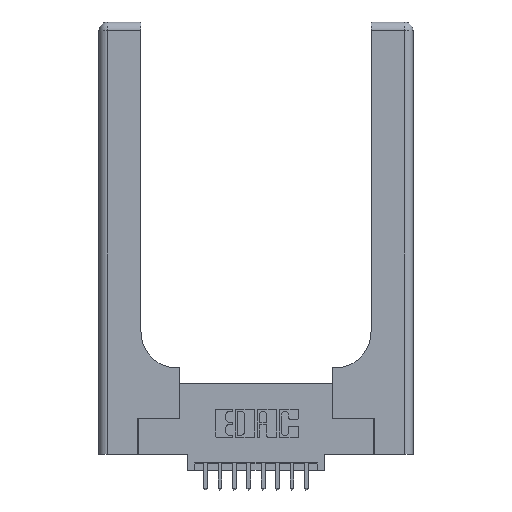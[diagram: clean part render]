
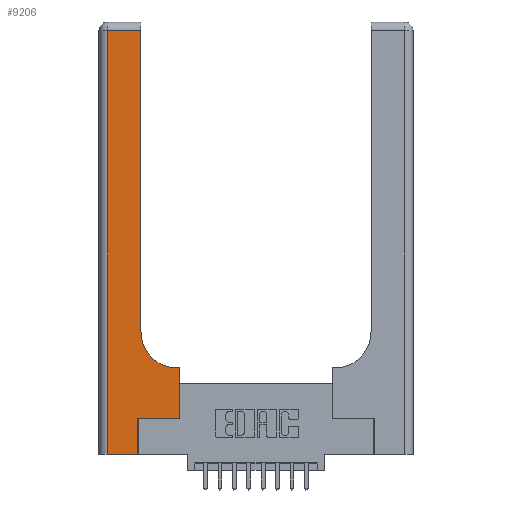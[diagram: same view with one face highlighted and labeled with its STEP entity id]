
A CAD part, top view. The second image highlights one B-rep face of the part: STEP entity #9206.
In plain terms, the highlighted planar face has unit normal (0, 0, 1).
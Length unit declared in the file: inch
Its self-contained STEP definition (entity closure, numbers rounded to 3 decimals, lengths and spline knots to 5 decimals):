
#89 = VERTEX_POINT ( 'NONE', #3098 ) ;
#274 = EDGE_CURVE ( 'NONE', #4211, #10207, #3985, .T. ) ;
#638 = VECTOR ( 'NONE', #4771, 39.37008 ) ;
#781 = LINE ( 'NONE', #11158, #16018 ) ;
#906 = FACE_OUTER_BOUND ( 'NONE', #12245, .T. ) ;
#949 = ORIENTED_EDGE ( 'NONE', *, *, #274, .T. ) ;
#1540 = ORIENTED_EDGE ( 'NONE', *, *, #3682, .T. ) ;
#1818 = DIRECTION ( 'NONE',  ( -1., 0., 0. ) ) ;
#2000 = VECTOR ( 'NONE', #11698, 39.37008 ) ;
#2294 = EDGE_CURVE ( 'NONE', #89, #9336, #5552, .T. ) ;
#2341 = LINE ( 'NONE', #11331, #15813 ) ;
#2592 = LINE ( 'NONE', #10389, #2000 ) ;
#3098 = CARTESIAN_POINT ( 'NONE',  ( 0.06, 2.94, 0.37 ) ) ;
#3407 = VECTOR ( 'NONE', #9392, 39.37008 ) ;
#3682 = EDGE_CURVE ( 'NONE', #9336, #14236, #8058, .T. ) ;
#3825 = CARTESIAN_POINT ( 'NONE',  ( 0.5585, 0.25, 0.37 ) ) ;
#3893 = AXIS2_PLACEMENT_3D ( 'NONE', #16119, #11271, #12535 ) ;
#3985 = CIRCLE ( 'NONE', #3893, 0.25 ) ;
#4026 = CARTESIAN_POINT ( 'NONE',  ( 0.269, 0.25, 0.37 ) ) ;
#4211 = VERTEX_POINT ( 'NONE', #8186 ) ;
#4319 = PLANE ( 'NONE',  #9111 ) ;
#4596 = DIRECTION ( 'NONE',  ( 0., 1., 0. ) ) ;
#4752 = EDGE_CURVE ( 'NONE', #10694, #9421, #10608, .T. ) ;
#4771 = DIRECTION ( 'NONE',  ( 1., 0., 0. ) ) ;
#4929 = CARTESIAN_POINT ( 'NONE',  ( 0.2915, 0.85, 0.37 ) ) ;
#5077 = ORIENTED_EDGE ( 'NONE', *, *, #10045, .T. ) ;
#5552 = LINE ( 'NONE', #13077, #3407 ) ;
#5838 = CARTESIAN_POINT ( 'NONE',  ( 0.5585, 0.6, 0.37 ) ) ;
#6162 = EDGE_CURVE ( 'NONE', #10207, #9339, #2341, .T. ) ;
#6340 = VECTOR ( 'NONE', #1818, 39.37008 ) ;
#7088 = CARTESIAN_POINT ( 'NONE',  ( 0., 3., 0.37 ) ) ;
#8058 = LINE ( 'NONE', #10932, #638 ) ;
#8186 = CARTESIAN_POINT ( 'NONE',  ( 0.5415, 0.6, 0.37 ) ) ;
#8373 = LINE ( 'NONE', #10858, #8581 ) ;
#8428 = ORIENTED_EDGE ( 'NONE', *, *, #14987, .T. ) ;
#8581 = VECTOR ( 'NONE', #4596, 39.37008 ) ;
#8621 = ORIENTED_EDGE ( 'NONE', *, *, #13351, .T. ) ;
#8641 = CARTESIAN_POINT ( 'NONE',  ( 0.06, 0., 0.37 ) ) ;
#9111 = AXIS2_PLACEMENT_3D ( 'NONE', #7088, #14556, #14493 ) ;
#9206 = ADVANCED_FACE ( 'NONE', ( #906 ), #4319, .F. ) ;
#9336 = VERTEX_POINT ( 'NONE', #8641 ) ;
#9339 = VERTEX_POINT ( 'NONE', #12603 ) ;
#9392 = DIRECTION ( 'NONE',  ( 0., -1., 0. ) ) ;
#9421 = VERTEX_POINT ( 'NONE', #5838 ) ;
#9455 = ORIENTED_EDGE ( 'NONE', *, *, #6162, .T. ) ;
#10045 = EDGE_CURVE ( 'NONE', #9339, #89, #12041, .T. ) ;
#10207 = VERTEX_POINT ( 'NONE', #4929 ) ;
#10389 = CARTESIAN_POINT ( 'NONE',  ( 0.269, 0.25, 0.37 ) ) ;
#10608 = LINE ( 'NONE', #3825, #15474 ) ;
#10673 = CARTESIAN_POINT ( 'NONE',  ( 0.269, 0., 0.37 ) ) ;
#10694 = VERTEX_POINT ( 'NONE', #14426 ) ;
#10858 = CARTESIAN_POINT ( 'NONE',  ( 0.269, 0., 0.37 ) ) ;
#10932 = CARTESIAN_POINT ( 'NONE',  ( 0., 0., 0.37 ) ) ;
#11158 = CARTESIAN_POINT ( 'NONE',  ( 0.2915, 0.6, 0.37 ) ) ;
#11271 = DIRECTION ( 'NONE',  ( 0., 0., -1. ) ) ;
#11331 = CARTESIAN_POINT ( 'NONE',  ( 0.2915, 3., 0.37 ) ) ;
#11698 = DIRECTION ( 'NONE',  ( 1., 0., 0. ) ) ;
#11811 = VERTEX_POINT ( 'NONE', #4026 ) ;
#11813 = CARTESIAN_POINT ( 'NONE',  ( 0., 2.94, 0.37 ) ) ;
#11949 = EDGE_CURVE ( 'NONE', #11811, #10694, #2592, .T. ) ;
#12041 = LINE ( 'NONE', #11813, #6340 ) ;
#12245 = EDGE_LOOP ( 'NONE', ( #9455, #5077, #12972, #1540, #8428, #12641, #13199, #8621, #949 ) ) ;
#12535 = DIRECTION ( 'NONE',  ( 1., 0., 0. ) ) ;
#12603 = CARTESIAN_POINT ( 'NONE',  ( 0.2915, 2.94, 0.37 ) ) ;
#12641 = ORIENTED_EDGE ( 'NONE', *, *, #11949, .T. ) ;
#12802 = DIRECTION ( 'NONE',  ( 0., 1., 0. ) ) ;
#12972 = ORIENTED_EDGE ( 'NONE', *, *, #2294, .T. ) ;
#13077 = CARTESIAN_POINT ( 'NONE',  ( 0.06, 3., 0.37 ) ) ;
#13199 = ORIENTED_EDGE ( 'NONE', *, *, #4752, .T. ) ;
#13351 = EDGE_CURVE ( 'NONE', #9421, #4211, #781, .T. ) ;
#13898 = DIRECTION ( 'NONE',  ( 0., 1., 0. ) ) ;
#14236 = VERTEX_POINT ( 'NONE', #10673 ) ;
#14426 = CARTESIAN_POINT ( 'NONE',  ( 0.5585, 0.25, 0.37 ) ) ;
#14493 = DIRECTION ( 'NONE',  ( -1., 0., 0. ) ) ;
#14556 = DIRECTION ( 'NONE',  ( 0., 0., -1. ) ) ;
#14704 = DIRECTION ( 'NONE',  ( -1., 0., 0. ) ) ;
#14987 = EDGE_CURVE ( 'NONE', #14236, #11811, #8373, .T. ) ;
#15474 = VECTOR ( 'NONE', #13898, 39.37008 ) ;
#15813 = VECTOR ( 'NONE', #12802, 39.37008 ) ;
#16018 = VECTOR ( 'NONE', #14704, 39.37008 ) ;
#16119 = CARTESIAN_POINT ( 'NONE',  ( 0.5415, 0.85, 0.37 ) ) ;
